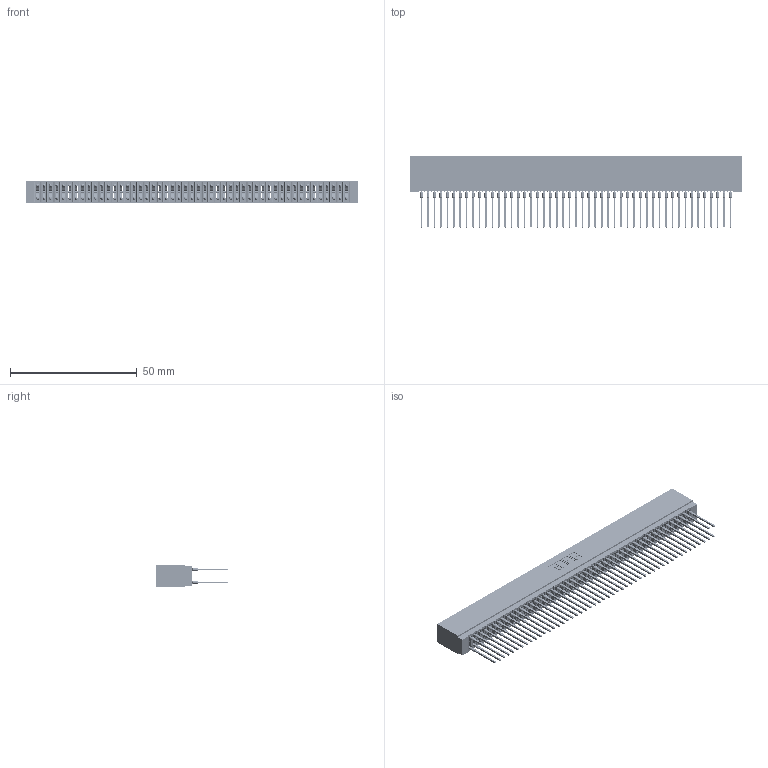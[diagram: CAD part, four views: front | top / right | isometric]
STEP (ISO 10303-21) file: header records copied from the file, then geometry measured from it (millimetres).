
FILE_DESCRIPTION (( 'STEP AP203' ), '1' );
FILE_NAME ('725-098-540-201.STEP', '2020-09-10T08:11:53', ( '' ), ( '' ), 'SwSTEP 2.0', 'SolidWorks 2020', '' );
FILE_SCHEMA (( 'CONFIG_CONTROL_DESIGN' ));
Length unit declared in the file: inch
Products named in the file (3): 725 Part_Insulator Option - 01; 745-292-001_540; 725-098-540-201
Assembly tree (99 placements, depth 2):
  725-098-540-201
    725 Part_Insulator Option - 01
    745-292-001_540  x98
Bounding box: 131.06 x 28.21 x 8.89 mm (x, y, z)
Volume: 10647.8 mm3; surface area: 23777.9 mm2
Topology: 99 solids, 99 shells, 8866 faces, 23823 edges, 14966 vertices
Faces by surface type: plane 4563, bspline 1960, cylinder 1755, torus 588
Entity records: 81507 total; most frequent: CARTESIAN_POINT 14635, ORIENTED_EDGE 14084, DIRECTION 12300, EDGE_CURVE 7042, LINE 6566, VECTOR 6566, VERTEX_POINT 4490, AXIS2_PLACEMENT_3D 2867
